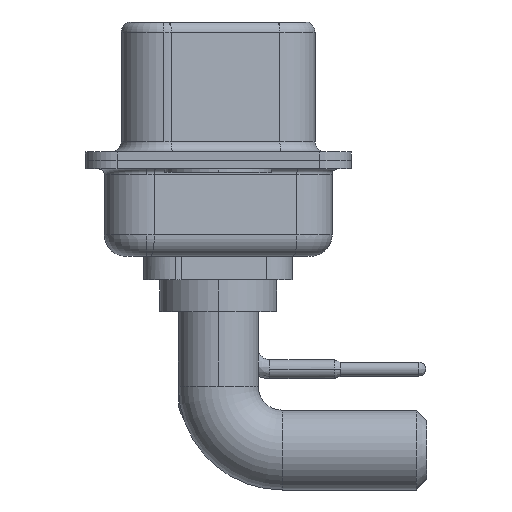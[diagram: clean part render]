
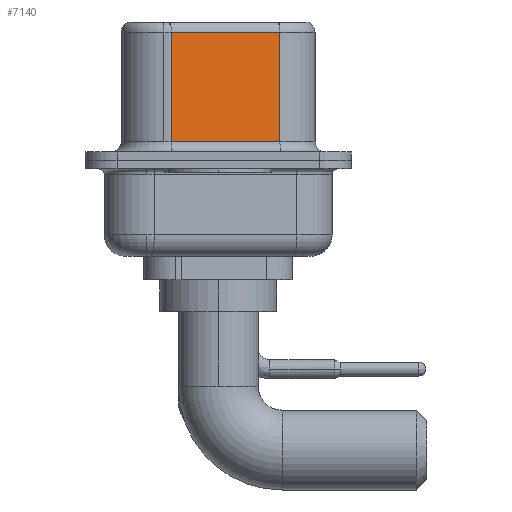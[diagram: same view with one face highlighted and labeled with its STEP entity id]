
A CAD part, left-side view. The second image highlights one B-rep face of the part: STEP entity #7140.
In plain terms, the highlighted planar face has unit normal (-0.985, -0.174, 0).
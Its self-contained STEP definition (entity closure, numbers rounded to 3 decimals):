
#57 = CARTESIAN_POINT ( 'NONE',  ( 4.58, -2.897, 0.9 ) ) ;
#617 = CARTESIAN_POINT ( 'NONE',  ( 4.58, -2.897, 6.02 ) ) ;
#726 = CARTESIAN_POINT ( 'NONE',  ( 3.68, 2.203, 0.9 ) ) ;
#1354 = CARTESIAN_POINT ( 'NONE',  ( 4.58, -2.897, 6.52 ) ) ;
#1792 = LINE ( 'NONE', #57, #13621 ) ;
#3017 = EDGE_CURVE ( 'NONE', #20153, #16334, #12909, .T. ) ;
#3355 = VECTOR ( 'NONE', #4509, 1000. ) ;
#3679 = ORIENTED_EDGE ( 'NONE', *, *, #4835, .T. ) ;
#4509 = DIRECTION ( 'NONE',  ( -0.174, 0.985, 0. ) ) ;
#4835 = EDGE_CURVE ( 'NONE', #20153, #6253, #18163, .T. ) ;
#5436 = EDGE_CURVE ( 'NONE', #7319, #16334, #1792, .T. ) ;
#6253 = VERTEX_POINT ( 'NONE', #6916 ) ;
#6916 = CARTESIAN_POINT ( 'NONE',  ( 3.68, 2.203, 6.02 ) ) ;
#7081 = DIRECTION ( 'NONE',  ( 0.174, -0.985, 0. ) ) ;
#7140 = ADVANCED_FACE ( 'NONE', ( #11686 ), #15122, .F. ) ;
#7319 = VERTEX_POINT ( 'NONE', #726 ) ;
#7934 = CARTESIAN_POINT ( 'NONE',  ( 3.68, 2.203, 6.52 ) ) ;
#8245 = ORIENTED_EDGE ( 'NONE', *, *, #5436, .T. ) ;
#8337 = AXIS2_PLACEMENT_3D ( 'NONE', #1354, #15242, #17074 ) ;
#9589 = EDGE_LOOP ( 'NONE', ( #19194, #3679, #12275, #8245 ) ) ;
#10964 = CARTESIAN_POINT ( 'NONE',  ( 4.58, -2.897, 6.52 ) ) ;
#11197 = DIRECTION ( 'NONE',  ( 0., 0., -1. ) ) ;
#11686 = FACE_OUTER_BOUND ( 'NONE', #9589, .T. ) ;
#12275 = ORIENTED_EDGE ( 'NONE', *, *, #18995, .T. ) ;
#12909 = LINE ( 'NONE', #10964, #19943 ) ;
#13621 = VECTOR ( 'NONE', #7081, 1000. ) ;
#14797 = DIRECTION ( 'NONE',  ( 0., 0., -1. ) ) ;
#15122 = PLANE ( 'NONE',  #8337 ) ;
#15242 = DIRECTION ( 'NONE',  ( 0.985, 0.174, 0. ) ) ;
#16134 = CARTESIAN_POINT ( 'NONE',  ( 4.58, -2.897, 0.9 ) ) ;
#16334 = VERTEX_POINT ( 'NONE', #16134 ) ;
#17074 = DIRECTION ( 'NONE',  ( -0.174, 0.985, 0. ) ) ;
#18163 = LINE ( 'NONE', #617, #3355 ) ;
#18348 = CARTESIAN_POINT ( 'NONE',  ( 4.58, -2.897, 6.02 ) ) ;
#18995 = EDGE_CURVE ( 'NONE', #6253, #7319, #20306, .T. ) ;
#19194 = ORIENTED_EDGE ( 'NONE', *, *, #3017, .F. ) ;
#19553 = VECTOR ( 'NONE', #14797, 1000. ) ;
#19943 = VECTOR ( 'NONE', #11197, 1000. ) ;
#20153 = VERTEX_POINT ( 'NONE', #18348 ) ;
#20306 = LINE ( 'NONE', #7934, #19553 ) ;
